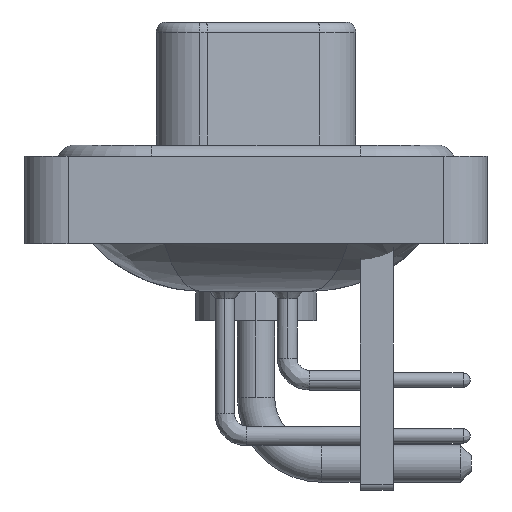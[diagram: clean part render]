
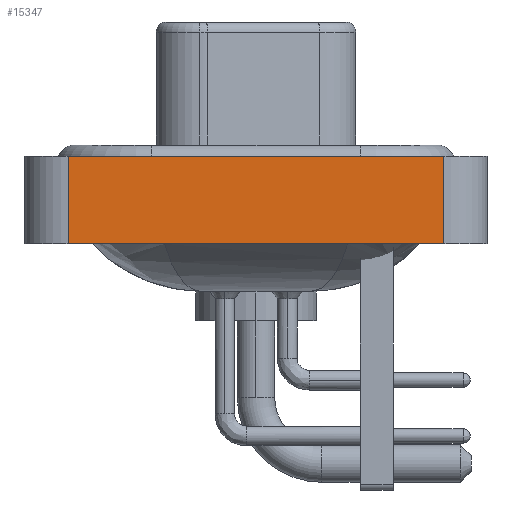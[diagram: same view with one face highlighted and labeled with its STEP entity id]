
A CAD part, left-side view. The second image highlights one B-rep face of the part: STEP entity #15347.
In plain terms, the highlighted planar face has unit normal (-1, 0, 0).
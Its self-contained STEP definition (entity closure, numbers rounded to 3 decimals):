
#55 = LINE ( 'NONE', #9733, #25462 ) ;
#2023 = LINE ( 'NONE', #28382, #12682 ) ;
#2823 = AXIS2_PLACEMENT_3D ( 'NONE', #5789, #27086, #15155 ) ;
#3339 = CARTESIAN_POINT ( 'NONE',  ( -7.35, 8.55, 0.4 ) ) ;
#4518 = CARTESIAN_POINT ( 'NONE',  ( -7.35, -8.55, -3.6 ) ) ;
#5789 = CARTESIAN_POINT ( 'NONE',  ( -7.35, -8.55, -3.6 ) ) ;
#7194 = EDGE_CURVE ( 'NONE', #26995, #14077, #27974, .T. ) ;
#8239 = PLANE ( 'NONE',  #2823 ) ;
#9733 = CARTESIAN_POINT ( 'NONE',  ( -7.35, 8.55, -3.6 ) ) ;
#10085 = VECTOR ( 'NONE', #11428, 1000. ) ;
#10380 = ORIENTED_EDGE ( 'NONE', *, *, #22343, .F. ) ;
#11378 = DIRECTION ( 'NONE',  ( 0., -1., 0. ) ) ;
#11428 = DIRECTION ( 'NONE',  ( 0., 0., 1. ) ) ;
#11778 = ORIENTED_EDGE ( 'NONE', *, *, #18446, .F. ) ;
#12682 = VECTOR ( 'NONE', #11378, 1000. ) ;
#14077 = VERTEX_POINT ( 'NONE', #24086 ) ;
#15014 = DIRECTION ( 'NONE',  ( 0., -1., 0. ) ) ;
#15155 = DIRECTION ( 'NONE',  ( 0., 0., 1. ) ) ;
#15162 = EDGE_CURVE ( 'NONE', #21915, #26995, #2023, .T. ) ;
#15347 = ADVANCED_FACE ( 'NONE', ( #22332 ), #8239, .T. ) ;
#16821 = CARTESIAN_POINT ( 'NONE',  ( -7.35, 8.55, -3.6 ) ) ;
#17101 = VERTEX_POINT ( 'NONE', #3339 ) ;
#18249 = EDGE_LOOP ( 'NONE', ( #29382, #11778, #10380, #26953 ) ) ;
#18446 = EDGE_CURVE ( 'NONE', #17101, #14077, #19595, .T. ) ;
#18862 = VECTOR ( 'NONE', #15014, 1000. ) ;
#18948 = DIRECTION ( 'NONE',  ( 0., 0., 1. ) ) ;
#19595 = LINE ( 'NONE', #24022, #18862 ) ;
#20397 = CARTESIAN_POINT ( 'NONE',  ( -7.35, -8.55, -3.6 ) ) ;
#21915 = VERTEX_POINT ( 'NONE', #16821 ) ;
#22332 = FACE_OUTER_BOUND ( 'NONE', #18249, .T. ) ;
#22343 = EDGE_CURVE ( 'NONE', #21915, #17101, #55, .T. ) ;
#24022 = CARTESIAN_POINT ( 'NONE',  ( -7.35, -8.55, 0.4 ) ) ;
#24086 = CARTESIAN_POINT ( 'NONE',  ( -7.35, -8.55, 0.4 ) ) ;
#25462 = VECTOR ( 'NONE', #18948, 1000. ) ;
#26953 = ORIENTED_EDGE ( 'NONE', *, *, #15162, .T. ) ;
#26995 = VERTEX_POINT ( 'NONE', #20397 ) ;
#27086 = DIRECTION ( 'NONE',  ( -1., 0., 0. ) ) ;
#27974 = LINE ( 'NONE', #4518, #10085 ) ;
#28382 = CARTESIAN_POINT ( 'NONE',  ( -7.35, -8.55, -3.6 ) ) ;
#29382 = ORIENTED_EDGE ( 'NONE', *, *, #7194, .T. ) ;
